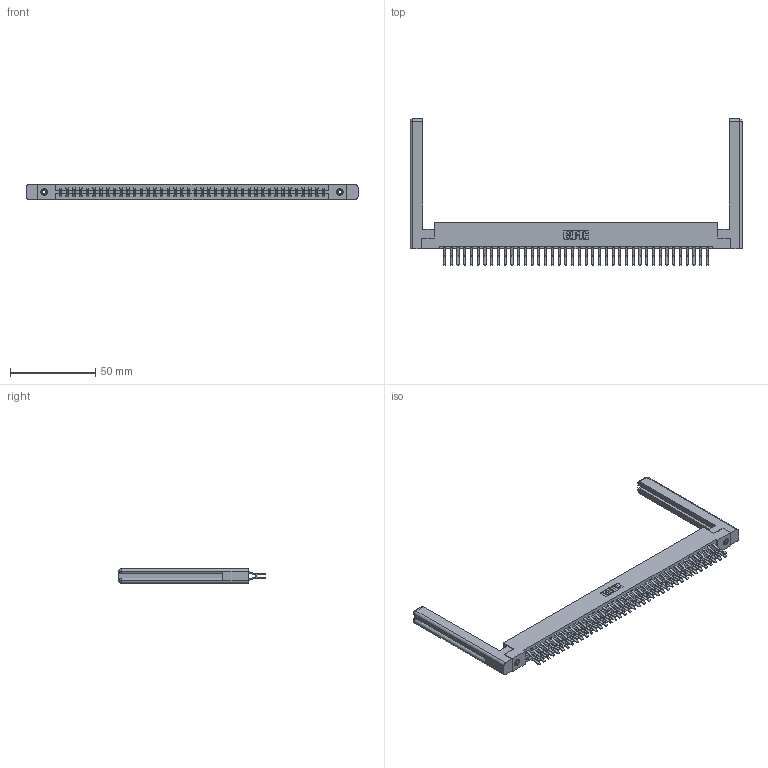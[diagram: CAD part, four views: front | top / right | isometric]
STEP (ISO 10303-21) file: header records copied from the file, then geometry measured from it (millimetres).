
FILE_DESCRIPTION (( 'STEP AP203' ), '1' );
FILE_NAME ('337-080-560-258.STEP', '2019-10-10T12:40:42', ( '' ), ( '' ), 'SwSTEP 2.0', 'SolidWorks 2016', '' );
FILE_SCHEMA (( 'CONFIG_CONTROL_DESIGN' ));
Length unit declared in the file: inch
Products named in the file (5): 307-220-058; 345-250-001_345-250-001-102; 345-292-001_560 Tail; 337 Part_Flush Mounting Lugs - 0.156 Dia-TI; 337-080-560-258
Assembly tree (85 placements, depth 2):
  337-080-560-258
    337 Part_Flush Mounting Lugs - 0.156 Dia-TI
    345-292-001_560 Tail  x80
    345-250-001_345-250-001-102  x2
    307-220-058  x2
Bounding box: 195.12 x 85.87 x 9.4 mm (x, y, z)
Volume: 28203.7 mm3; surface area: 30354.9 mm2
Topology: 85 solids, 85 shells, 4736 faces, 14025 edges, 9230 vertices
Faces by surface type: plane 3194, cylinder 1518, cone 12, torus 12
Entity records: 33994 total; most frequent: CARTESIAN_POINT 5737, ORIENTED_EDGE 5612, DIRECTION 4902, EDGE_CURVE 2806, LINE 2626, VECTOR 2626, VERTEX_POINT 1862, AXIS2_PLACEMENT_3D 1138
